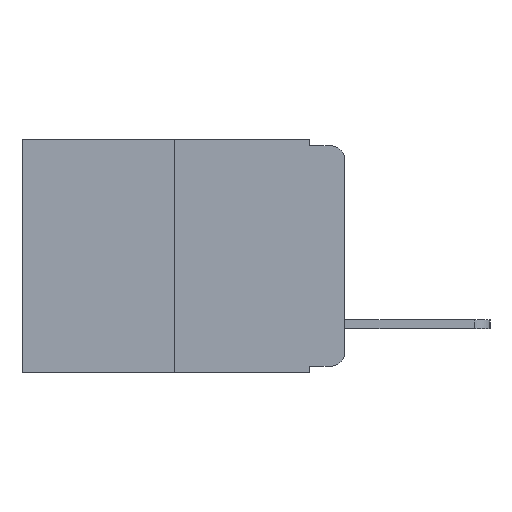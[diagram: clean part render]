
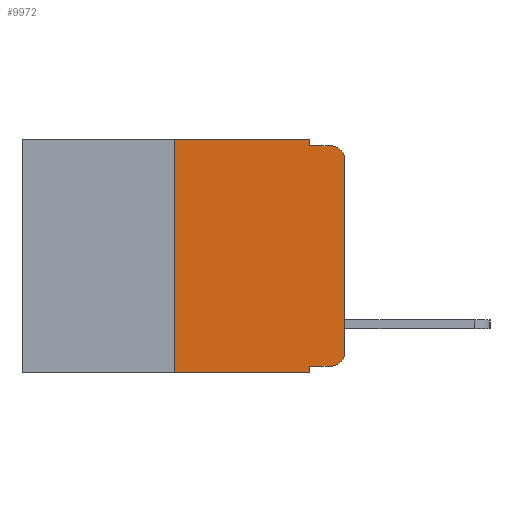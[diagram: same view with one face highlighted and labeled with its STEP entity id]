
A CAD part, left-side view. The second image highlights one B-rep face of the part: STEP entity #9972.
In plain terms, the highlighted planar face has unit normal (-1, 0, 0).
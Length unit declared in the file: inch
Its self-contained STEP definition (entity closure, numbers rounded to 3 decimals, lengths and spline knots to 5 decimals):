
#110 = ORIENTED_EDGE ( 'NONE', *, *, #1844, .T. ) ;
#273 = VERTEX_POINT ( 'NONE', #11521 ) ;
#610 = CARTESIAN_POINT ( 'NONE',  ( 0., 0.473, 0. ) ) ;
#762 = DIRECTION ( 'NONE',  ( 0., -1., 0. ) ) ;
#796 = VECTOR ( 'NONE', #2132, 39.37008 ) ;
#904 = VERTEX_POINT ( 'NONE', #9935 ) ;
#1053 = EDGE_LOOP ( 'NONE', ( #110, #1539, #5935, #6486, #4110, #3771, #3025, #8420, #10488, #6539 ) ) ;
#1187 = VERTEX_POINT ( 'NONE', #3215 ) ;
#1323 = VERTEX_POINT ( 'NONE', #6303 ) ;
#1501 = CARTESIAN_POINT ( 'NONE',  ( 0., 0.051, 0. ) ) ;
#1539 = ORIENTED_EDGE ( 'NONE', *, *, #1766, .T. ) ;
#1581 = DIRECTION ( 'NONE',  ( 0., 0., -1. ) ) ;
#1748 = CARTESIAN_POINT ( 'NONE',  ( 0., 0.25, 0. ) ) ;
#1766 = EDGE_CURVE ( 'NONE', #1323, #3240, #6141, .T. ) ;
#1844 = EDGE_CURVE ( 'NONE', #904, #1323, #3448, .T. ) ;
#1930 = VERTEX_POINT ( 'NONE', #8245 ) ;
#2073 = CARTESIAN_POINT ( 'NONE',  ( 0., 0.051, 0. ) ) ;
#2098 = EDGE_CURVE ( 'NONE', #273, #11092, #5153, .T. ) ;
#2132 = DIRECTION ( 'NONE',  ( 0., -1., 0. ) ) ;
#2458 = CARTESIAN_POINT ( 'NONE',  ( 0., 0.051, -0.01 ) ) ;
#2461 = DIRECTION ( 'NONE',  ( 0., 0., -1. ) ) ;
#3025 = ORIENTED_EDGE ( 'NONE', *, *, #11033, .T. ) ;
#3206 = VERTEX_POINT ( 'NONE', #9524 ) ;
#3215 = CARTESIAN_POINT ( 'NONE',  ( 0., 0.25, -0.343 ) ) ;
#3240 = VERTEX_POINT ( 'NONE', #8228 ) ;
#3266 = CARTESIAN_POINT ( 'NONE',  ( 0., 0.051, -0.333 ) ) ;
#3282 = CIRCLE ( 'NONE', #7611, 0.02 ) ;
#3339 = LINE ( 'NONE', #2458, #796 ) ;
#3448 = LINE ( 'NONE', #11059, #5293 ) ;
#3551 = DIRECTION ( 'NONE',  ( 0., -1., 0. ) ) ;
#3771 = ORIENTED_EDGE ( 'NONE', *, *, #4986, .F. ) ;
#4110 = ORIENTED_EDGE ( 'NONE', *, *, #4114, .F. ) ;
#4114 = EDGE_CURVE ( 'NONE', #4937, #3206, #7183, .T. ) ;
#4316 = VECTOR ( 'NONE', #8428, 39.37008 ) ;
#4937 = VERTEX_POINT ( 'NONE', #1748 ) ;
#4986 = EDGE_CURVE ( 'NONE', #1187, #4937, #11522, .T. ) ;
#5121 = EDGE_CURVE ( 'NONE', #8775, #3240, #3339, .T. ) ;
#5153 = LINE ( 'NONE', #3266, #5439 ) ;
#5226 = CARTESIAN_POINT ( 'NONE',  ( 0., 0.02, -0.313 ) ) ;
#5234 = CARTESIAN_POINT ( 'NONE',  ( 0., 0.051, -0.01 ) ) ;
#5285 = PLANE ( 'NONE',  #6818 ) ;
#5293 = VECTOR ( 'NONE', #11034, 39.37008 ) ;
#5439 = VECTOR ( 'NONE', #3551, 39.37008 ) ;
#5935 = ORIENTED_EDGE ( 'NONE', *, *, #5121, .F. ) ;
#5977 = CARTESIAN_POINT ( 'NONE',  ( 0., 0.02, -0.333 ) ) ;
#6131 = DIRECTION ( 'NONE',  ( 0., 0., -1. ) ) ;
#6141 = CIRCLE ( 'NONE', #7644, 0.02 ) ;
#6303 = CARTESIAN_POINT ( 'NONE',  ( 0., 0., -0.03 ) ) ;
#6486 = ORIENTED_EDGE ( 'NONE', *, *, #8496, .F. ) ;
#6539 = ORIENTED_EDGE ( 'NONE', *, *, #7360, .T. ) ;
#6796 = FACE_OUTER_BOUND ( 'NONE', #1053, .T. ) ;
#6818 = AXIS2_PLACEMENT_3D ( 'NONE', #610, #7080, #1581 ) ;
#6828 = DIRECTION ( 'NONE',  ( 0., -1., 0. ) ) ;
#6884 = VECTOR ( 'NONE', #11650, 39.37008 ) ;
#7080 = DIRECTION ( 'NONE',  ( 1., 0., 0. ) ) ;
#7183 = LINE ( 'NONE', #7618, #7452 ) ;
#7350 = LINE ( 'NONE', #1501, #11706 ) ;
#7360 = EDGE_CURVE ( 'NONE', #11092, #904, #3282, .T. ) ;
#7452 = VECTOR ( 'NONE', #762, 39.37008 ) ;
#7611 = AXIS2_PLACEMENT_3D ( 'NONE', #5226, #11369, #6131 ) ;
#7618 = CARTESIAN_POINT ( 'NONE',  ( 0., 0.473, 0. ) ) ;
#7644 = AXIS2_PLACEMENT_3D ( 'NONE', #8181, #8167, #10401 ) ;
#8167 = DIRECTION ( 'NONE',  ( -1., 0., 0. ) ) ;
#8181 = CARTESIAN_POINT ( 'NONE',  ( 0., 0.02, -0.03 ) ) ;
#8228 = CARTESIAN_POINT ( 'NONE',  ( 0., 0.02, -0.01 ) ) ;
#8245 = CARTESIAN_POINT ( 'NONE',  ( 0., 0.051, -0.343 ) ) ;
#8420 = ORIENTED_EDGE ( 'NONE', *, *, #9936, .F. ) ;
#8428 = DIRECTION ( 'NONE',  ( 0., 0., -1. ) ) ;
#8496 = EDGE_CURVE ( 'NONE', #3206, #8775, #8751, .T. ) ;
#8751 = LINE ( 'NONE', #2073, #4316 ) ;
#8775 = VERTEX_POINT ( 'NONE', #5234 ) ;
#9501 = VECTOR ( 'NONE', #6828, 39.37008 ) ;
#9524 = CARTESIAN_POINT ( 'NONE',  ( 0., 0.051, 0. ) ) ;
#9935 = CARTESIAN_POINT ( 'NONE',  ( 0., 0., -0.313 ) ) ;
#9936 = EDGE_CURVE ( 'NONE', #273, #1930, #7350, .T. ) ;
#9972 = ADVANCED_FACE ( 'NONE', ( #6796 ), #5285, .F. ) ;
#10401 = DIRECTION ( 'NONE',  ( 0., 0., -1. ) ) ;
#10488 = ORIENTED_EDGE ( 'NONE', *, *, #2098, .T. ) ;
#11033 = EDGE_CURVE ( 'NONE', #1187, #1930, #11545, .T. ) ;
#11034 = DIRECTION ( 'NONE',  ( 0., 0., 1. ) ) ;
#11059 = CARTESIAN_POINT ( 'NONE',  ( 0., 0., 0. ) ) ;
#11092 = VERTEX_POINT ( 'NONE', #5977 ) ;
#11179 = CARTESIAN_POINT ( 'NONE',  ( 0., 0.473, -0.343 ) ) ;
#11369 = DIRECTION ( 'NONE',  ( -1., 0., 0. ) ) ;
#11521 = CARTESIAN_POINT ( 'NONE',  ( 0., 0.051, -0.333 ) ) ;
#11522 = LINE ( 'NONE', #11692, #6884 ) ;
#11545 = LINE ( 'NONE', #11179, #9501 ) ;
#11650 = DIRECTION ( 'NONE',  ( 0., 0., 1. ) ) ;
#11692 = CARTESIAN_POINT ( 'NONE',  ( 0., 0.25, 0. ) ) ;
#11706 = VECTOR ( 'NONE', #2461, 39.37008 ) ;
